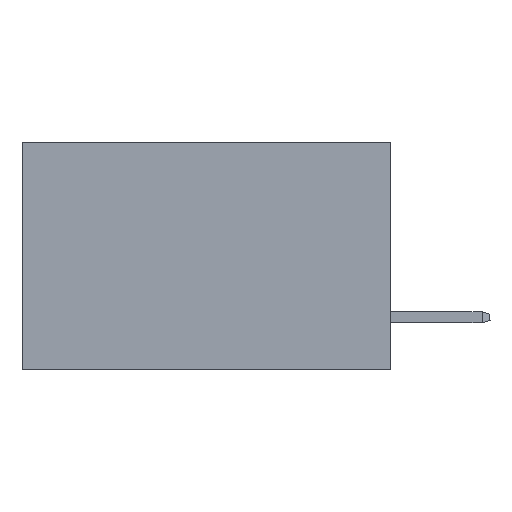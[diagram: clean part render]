
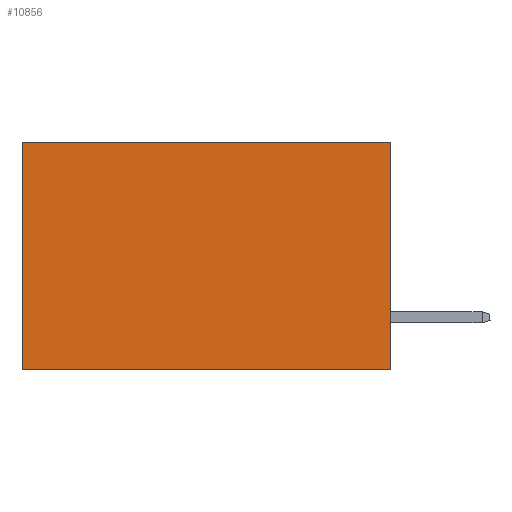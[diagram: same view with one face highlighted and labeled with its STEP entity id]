
A CAD part, left-side view. The second image highlights one B-rep face of the part: STEP entity #10856.
In plain terms, the highlighted planar face has unit normal (-1, 0, 0).
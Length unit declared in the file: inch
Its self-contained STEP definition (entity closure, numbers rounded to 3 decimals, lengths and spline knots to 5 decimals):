
#2047 = PLANE ( 'NONE',  #38172 ) ;
#2156 = VECTOR ( 'NONE', #6599, 39.37008 ) ;
#2297 = CARTESIAN_POINT ( 'NONE',  ( 0.2875, 0., 0. ) ) ;
#2378 = CARTESIAN_POINT ( 'NONE',  ( 0.2875, 0.6, 0. ) ) ;
#2574 = CARTESIAN_POINT ( 'NONE',  ( 0.2875, 0.6, 0. ) ) ;
#3420 = EDGE_CURVE ( 'NONE', #38526, #7559, #14979, .T. ) ;
#5952 = LINE ( 'NONE', #32342, #8568 ) ;
#6370 = ORIENTED_EDGE ( 'NONE', *, *, #19201, .T. ) ;
#6552 = VERTEX_POINT ( 'NONE', #20555 ) ;
#6599 = DIRECTION ( 'NONE',  ( 0., 0., -1. ) ) ;
#7559 = VERTEX_POINT ( 'NONE', #30009 ) ;
#8468 = EDGE_LOOP ( 'NONE', ( #8995, #24183, #32012, #6370 ) ) ;
#8568 = VECTOR ( 'NONE', #18590, 39.37008 ) ;
#8772 = DIRECTION ( 'NONE',  ( 0., 0., -1. ) ) ;
#8995 = ORIENTED_EDGE ( 'NONE', *, *, #3420, .T. ) ;
#10179 = DIRECTION ( 'NONE',  ( 0., 0., -1. ) ) ;
#10856 = ADVANCED_FACE ( 'NONE', ( #41945 ), #2047, .F. ) ;
#11095 = CARTESIAN_POINT ( 'NONE',  ( 0.2875, 0., -0.37 ) ) ;
#11142 = LINE ( 'NONE', #2297, #2156 ) ;
#13163 = DIRECTION ( 'NONE',  ( 1., 0., 0. ) ) ;
#14833 = VERTEX_POINT ( 'NONE', #11095 ) ;
#14979 = LINE ( 'NONE', #2378, #29794 ) ;
#18590 = DIRECTION ( 'NONE',  ( 0., 1., 0. ) ) ;
#19201 = EDGE_CURVE ( 'NONE', #6552, #38526, #22551, .T. ) ;
#20555 = CARTESIAN_POINT ( 'NONE',  ( 0.2875, 0., 0. ) ) ;
#22551 = LINE ( 'NONE', #23194, #41590 ) ;
#23194 = CARTESIAN_POINT ( 'NONE',  ( 0.2875, 0., 0. ) ) ;
#24183 = ORIENTED_EDGE ( 'NONE', *, *, #24649, .F. ) ;
#24649 = EDGE_CURVE ( 'NONE', #14833, #7559, #5952, .T. ) ;
#29794 = VECTOR ( 'NONE', #8772, 39.37008 ) ;
#30009 = CARTESIAN_POINT ( 'NONE',  ( 0.2875, 0.6, -0.37 ) ) ;
#32012 = ORIENTED_EDGE ( 'NONE', *, *, #32466, .F. ) ;
#32342 = CARTESIAN_POINT ( 'NONE',  ( 0.2875, 0., -0.37 ) ) ;
#32466 = EDGE_CURVE ( 'NONE', #6552, #14833, #11142, .T. ) ;
#35907 = CARTESIAN_POINT ( 'NONE',  ( 0.2875, 0., 0. ) ) ;
#38172 = AXIS2_PLACEMENT_3D ( 'NONE', #35907, #13163, #10179 ) ;
#38526 = VERTEX_POINT ( 'NONE', #2574 ) ;
#40219 = DIRECTION ( 'NONE',  ( 0., 1., 0. ) ) ;
#41590 = VECTOR ( 'NONE', #40219, 39.37008 ) ;
#41945 = FACE_OUTER_BOUND ( 'NONE', #8468, .T. ) ;
